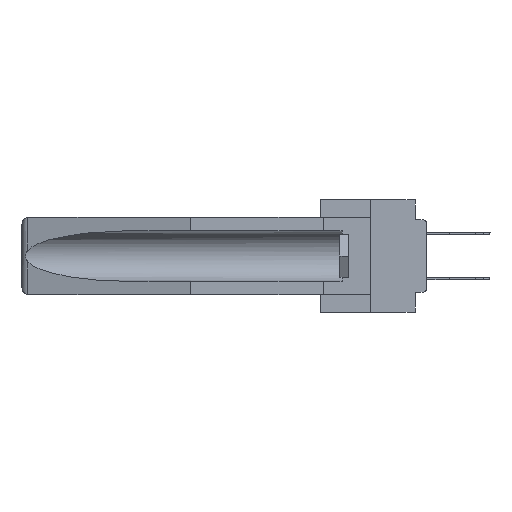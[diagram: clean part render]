
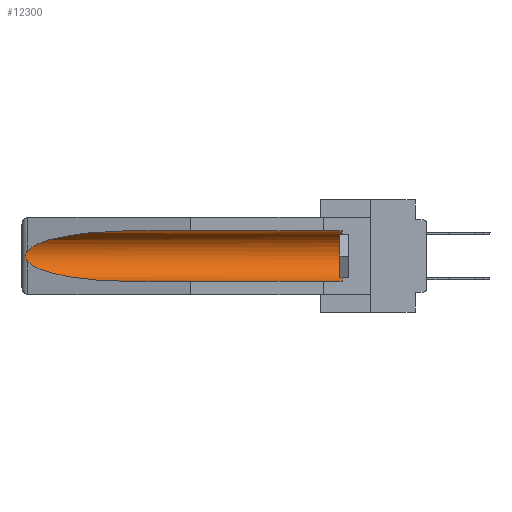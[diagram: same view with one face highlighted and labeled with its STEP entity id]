
A CAD part, left-side view. The second image highlights one B-rep face of the part: STEP entity #12300.
In plain terms, the highlighted cylindrical face has radius 2.857 mm (diameter 5.715 mm), a partial arc.
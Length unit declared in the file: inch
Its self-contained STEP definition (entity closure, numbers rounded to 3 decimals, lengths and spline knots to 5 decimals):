
#638 = EDGE_LOOP ( 'NONE', ( #1322, #2833, #20047, #8130, #3086, #2522 ) ) ;
#921 = VERTEX_POINT ( 'NONE', #11804 ) ;
#1167 = CARTESIAN_POINT ( 'NONE',  ( 0.155, 1.07973, -0.059 ) ) ;
#1322 = ORIENTED_EDGE ( 'NONE', *, *, #6234, .T. ) ;
#2012 = CARTESIAN_POINT ( 'NONE',  ( 0.26537, 1.52718, -0.19328 ) ) ;
#2322 = EDGE_CURVE ( 'NONE', #921, #24155, #18612, .T. ) ;
#2522 = ORIENTED_EDGE ( 'NONE', *, *, #7454, .T. ) ;
#2833 = ORIENTED_EDGE ( 'NONE', *, *, #29028, .T. ) ;
#2922 = DIRECTION ( 'NONE',  ( 0., 1., 0. ) ) ;
#3086 = ORIENTED_EDGE ( 'NONE', *, *, #18140, .T. ) ;
#3307 = AXIS2_PLACEMENT_3D ( 'NONE', #14580, #12378, #21364 ) ;
#4068 = CARTESIAN_POINT ( 'NONE',  ( 0.26537, 1.52718, -0.14972 ) ) ;
#4196 = CARTESIAN_POINT ( 'NONE',  ( 0.21114, 1.30732, -0.284 ) ) ;
#4208 = CARTESIAN_POINT ( 'NONE',  ( 0.26537, 1.52718, -0.19328 ) ) ;
#4729 = VECTOR ( 'NONE', #2922, 39.37008 ) ;
#5043 = VERTEX_POINT ( 'NONE', #19151 ) ;
#5595 = CYLINDRICAL_SURFACE ( 'NONE', #3307, 0.1125 ) ;
#6234 = EDGE_CURVE ( 'NONE', #28727, #5043, #13527, .T. ) ;
#7454 = EDGE_CURVE ( 'NONE', #21783, #28727, #16106, .T. ) ;
#8080 = CIRCLE ( 'NONE', #25982, 0.1125 ) ;
#8130 = ORIENTED_EDGE ( 'NONE', *, *, #12670, .F. ) ;
#8510 = CARTESIAN_POINT ( 'NONE',  ( 0.26597, 1.5296, -0.19026 ) ) ;
#8653 = CARTESIAN_POINT ( 'NONE',  ( 0.26654, 1.53092, -0.15636 ) ) ;
#10566 = CARTESIAN_POINT ( 'NONE',  ( 0.25451, 1.48313, -0.24835 ) ) ;
#10715 = CARTESIAN_POINT ( 'NONE',  ( 0.2675, 1.53308, -0.17534 ) ) ;
#11804 = CARTESIAN_POINT ( 'NONE',  ( 0.26537, 1.52718, -0.19328 ) ) ;
#11992 = CARTESIAN_POINT ( 'NONE',  ( 0.26537, 1.52718, -0.14972 ) ) ;
#12300 = ADVANCED_FACE ( 'NONE', ( #25782 ), #5595, .F. ) ;
#12378 = DIRECTION ( 'NONE',  ( 0., 1., 0. ) ) ;
#12670 = EDGE_CURVE ( 'NONE', #18982, #24155, #21332, .T. ) ;
#13527 =( BOUNDED_CURVE ( )  B_SPLINE_CURVE ( 3, ( #25691, #25824, #17119, #11992 ),
 .UNSPECIFIED., .F., .F. ) 
 B_SPLINE_CURVE_WITH_KNOTS ( ( 4, 4 ),
 ( 4.71239, 6.08839 ),
 .UNSPECIFIED. ) 
 CURVE ( )  GEOMETRIC_REPRESENTATION_ITEM ( )  RATIONAL_B_SPLINE_CURVE ( ( 1., 0.848, 0.848, 1. ) ) 
 REPRESENTATION_ITEM ( '' )  );
#13629 = CARTESIAN_POINT ( 'NONE',  ( 0.155, 1.07973, -0.284 ) ) ;
#13929 = B_SPLINE_CURVE_WITH_KNOTS ( 'NONE', 3,
 ( #4068, #23981, #8653, #19269, #26198, #10715, #19695, #28656, #8510, #4208 ),
 .UNSPECIFIED., .F., .F.,
 ( 4, 2, 2, 2, 4 ),
 ( 0., 0.00029, 0.00058, 0.00087, 0.00117 ),
 .UNSPECIFIED. ) ;
#14580 = CARTESIAN_POINT ( 'NONE',  ( 0.155, -0.30754, -0.1715 ) ) ;
#15504 = CARTESIAN_POINT ( 'NONE',  ( 0.155, 0.126, -0.1715 ) ) ;
#16106 = LINE ( 'NONE', #25403, #24719 ) ;
#17119 = CARTESIAN_POINT ( 'NONE',  ( 0.25451, 1.48313, -0.09465 ) ) ;
#18140 = EDGE_CURVE ( 'NONE', #18982, #21783, #8080, .T. ) ;
#18478 = DIRECTION ( 'NONE',  ( 0., 1., 0. ) ) ;
#18547 = CARTESIAN_POINT ( 'NONE',  ( 0.155, -0.30754, -0.284 ) ) ;
#18612 =( BOUNDED_CURVE ( )  B_SPLINE_CURVE ( 3, ( #2012, #10566, #4196, #19976 ),
 .UNSPECIFIED., .F., .F. ) 
 B_SPLINE_CURVE_WITH_KNOTS ( ( 4, 4 ),
 ( 0.1948, 1.5708 ),
 .UNSPECIFIED. ) 
 CURVE ( )  GEOMETRIC_REPRESENTATION_ITEM ( )  RATIONAL_B_SPLINE_CURVE ( ( 1., 0.848, 0.848, 1. ) ) 
 REPRESENTATION_ITEM ( '' )  );
#18982 = VERTEX_POINT ( 'NONE', #26617 ) ;
#19151 = CARTESIAN_POINT ( 'NONE',  ( 0.26537, 1.52718, -0.14972 ) ) ;
#19269 = CARTESIAN_POINT ( 'NONE',  ( 0.2673, 1.5327, -0.16383 ) ) ;
#19689 = CARTESIAN_POINT ( 'NONE',  ( 0.155, 0.126, -0.059 ) ) ;
#19695 = CARTESIAN_POINT ( 'NONE',  ( 0.2673, 1.53269, -0.17917 ) ) ;
#19976 = CARTESIAN_POINT ( 'NONE',  ( 0.155, 1.07973, -0.284 ) ) ;
#20047 = ORIENTED_EDGE ( 'NONE', *, *, #2322, .T. ) ;
#21332 = LINE ( 'NONE', #18547, #4729 ) ;
#21364 = DIRECTION ( 'NONE',  ( 0., 0., 1. ) ) ;
#21783 = VERTEX_POINT ( 'NONE', #19689 ) ;
#22296 = DIRECTION ( 'NONE',  ( 0., 0., 1. ) ) ;
#23981 = CARTESIAN_POINT ( 'NONE',  ( 0.26597, 1.52961, -0.15275 ) ) ;
#24155 = VERTEX_POINT ( 'NONE', #13629 ) ;
#24719 = VECTOR ( 'NONE', #18478, 39.37008 ) ;
#25403 = CARTESIAN_POINT ( 'NONE',  ( 0.155, -0.30754, -0.059 ) ) ;
#25691 = CARTESIAN_POINT ( 'NONE',  ( 0.155, 1.07973, -0.059 ) ) ;
#25782 = FACE_OUTER_BOUND ( 'NONE', #638, .T. ) ;
#25824 = CARTESIAN_POINT ( 'NONE',  ( 0.21114, 1.30732, -0.059 ) ) ;
#25982 = AXIS2_PLACEMENT_3D ( 'NONE', #15504, #28896, #22296 ) ;
#26198 = CARTESIAN_POINT ( 'NONE',  ( 0.2675, 1.53308, -0.16763 ) ) ;
#26617 = CARTESIAN_POINT ( 'NONE',  ( 0.155, 0.126, -0.284 ) ) ;
#28656 = CARTESIAN_POINT ( 'NONE',  ( 0.26655, 1.53094, -0.18657 ) ) ;
#28727 = VERTEX_POINT ( 'NONE', #1167 ) ;
#28896 = DIRECTION ( 'NONE',  ( 0., -1., 0. ) ) ;
#29028 = EDGE_CURVE ( 'NONE', #5043, #921, #13929, .T. ) ;
